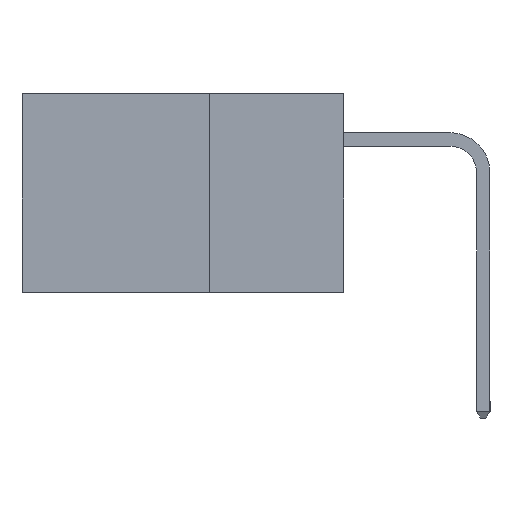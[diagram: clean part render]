
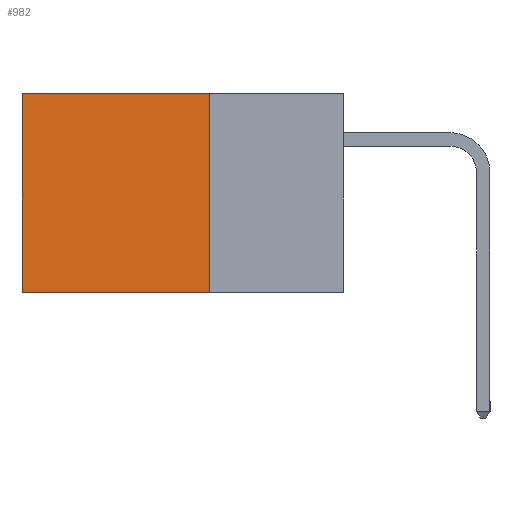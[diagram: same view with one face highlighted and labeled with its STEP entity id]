
A CAD part, left-side view. The second image highlights one B-rep face of the part: STEP entity #982.
In plain terms, the highlighted planar face has unit normal (-1, 0, 0).
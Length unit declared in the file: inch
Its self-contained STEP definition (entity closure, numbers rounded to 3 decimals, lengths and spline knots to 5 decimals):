
#306 = CARTESIAN_POINT ( 'NONE',  ( 0.2615, 0.6, -0.37 ) ) ;
#837 = CARTESIAN_POINT ( 'NONE',  ( 0.2615, 0.25, -0.37 ) ) ;
#886 = VECTOR ( 'NONE', #10595, 39.37008 ) ;
#982 = ADVANCED_FACE ( 'NONE', ( #10402 ), #11421, .F. ) ;
#1329 = LINE ( 'NONE', #6732, #9297 ) ;
#1463 = VERTEX_POINT ( 'NONE', #8787 ) ;
#1614 = CARTESIAN_POINT ( 'NONE',  ( 0.2615, 0.25, 0. ) ) ;
#2085 = DIRECTION ( 'NONE',  ( 1., 0., 0. ) ) ;
#2763 = VECTOR ( 'NONE', #12328, 39.37008 ) ;
#2825 = CARTESIAN_POINT ( 'NONE',  ( 0.2615, 0.25, -0.37 ) ) ;
#3393 = DIRECTION ( 'NONE',  ( 0., 0., -1. ) ) ;
#3701 = ORIENTED_EDGE ( 'NONE', *, *, #11272, .T. ) ;
#5137 = ORIENTED_EDGE ( 'NONE', *, *, #6116, .F. ) ;
#5272 = EDGE_LOOP ( 'NONE', ( #3701, #8729, #5137, #11553 ) ) ;
#5553 = EDGE_CURVE ( 'NONE', #11752, #8495, #1329, .T. ) ;
#5576 = CARTESIAN_POINT ( 'NONE',  ( 0.2615, 0.25, -0.37 ) ) ;
#6094 = VERTEX_POINT ( 'NONE', #2825 ) ;
#6116 = EDGE_CURVE ( 'NONE', #11752, #6094, #9096, .T. ) ;
#6179 = LINE ( 'NONE', #7019, #7090 ) ;
#6732 = CARTESIAN_POINT ( 'NONE',  ( 0.2615, 0.25, 0. ) ) ;
#6882 = DIRECTION ( 'NONE',  ( 0., 1., 0. ) ) ;
#7019 = CARTESIAN_POINT ( 'NONE',  ( 0.2615, 0.25, -0.37 ) ) ;
#7090 = VECTOR ( 'NONE', #11550, 39.37008 ) ;
#7552 = EDGE_CURVE ( 'NONE', #6094, #1463, #6179, .T. ) ;
#8495 = VERTEX_POINT ( 'NONE', #11312 ) ;
#8654 = AXIS2_PLACEMENT_3D ( 'NONE', #5576, #2085, #3393 ) ;
#8729 = ORIENTED_EDGE ( 'NONE', *, *, #7552, .F. ) ;
#8787 = CARTESIAN_POINT ( 'NONE',  ( 0.2615, 0.6, -0.37 ) ) ;
#9096 = LINE ( 'NONE', #837, #2763 ) ;
#9297 = VECTOR ( 'NONE', #6882, 39.37008 ) ;
#10402 = FACE_OUTER_BOUND ( 'NONE', #5272, .T. ) ;
#10595 = DIRECTION ( 'NONE',  ( 0., 0., -1. ) ) ;
#11272 = EDGE_CURVE ( 'NONE', #8495, #1463, #14585, .T. ) ;
#11312 = CARTESIAN_POINT ( 'NONE',  ( 0.2615, 0.6, 0. ) ) ;
#11421 = PLANE ( 'NONE',  #8654 ) ;
#11550 = DIRECTION ( 'NONE',  ( 0., 1., 0. ) ) ;
#11553 = ORIENTED_EDGE ( 'NONE', *, *, #5553, .T. ) ;
#11752 = VERTEX_POINT ( 'NONE', #1614 ) ;
#12328 = DIRECTION ( 'NONE',  ( 0., 0., -1. ) ) ;
#14585 = LINE ( 'NONE', #306, #886 ) ;
